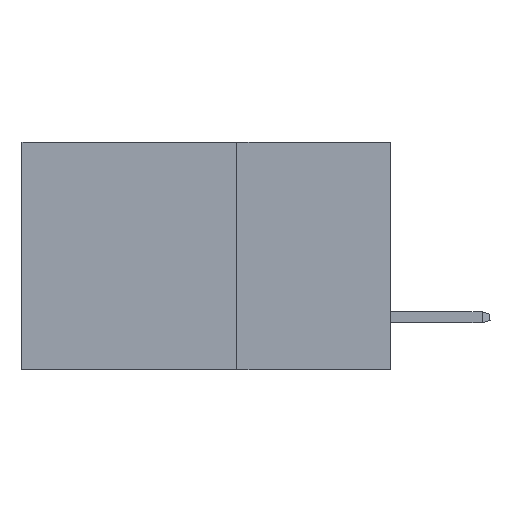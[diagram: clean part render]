
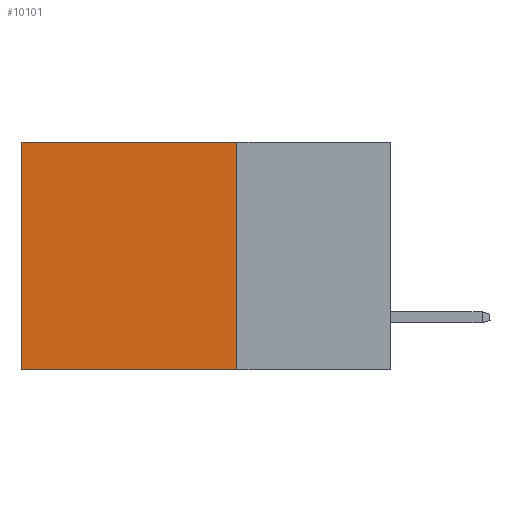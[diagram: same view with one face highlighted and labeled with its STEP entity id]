
A CAD part, left-side view. The second image highlights one B-rep face of the part: STEP entity #10101.
In plain terms, the highlighted planar face has unit normal (-1, 0, 0).
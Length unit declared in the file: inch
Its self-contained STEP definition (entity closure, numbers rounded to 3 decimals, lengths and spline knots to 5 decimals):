
#240 = ORIENTED_EDGE ( 'NONE', *, *, #2919, .T. ) ;
#477 = EDGE_LOOP ( 'NONE', ( #240, #1114, #8735, #3620 ) ) ;
#1114 = ORIENTED_EDGE ( 'NONE', *, *, #8586, .F. ) ;
#1245 = DIRECTION ( 'NONE',  ( 1., 0., 0. ) ) ;
#1264 = VECTOR ( 'NONE', #7803, 39.37008 ) ;
#1286 = PLANE ( 'NONE',  #10091 ) ;
#1387 = EDGE_CURVE ( 'NONE', #11843, #10115, #9545, .T. ) ;
#1590 = CARTESIAN_POINT ( 'NONE',  ( 0.2875, 0.25, -0.37 ) ) ;
#1961 = DIRECTION ( 'NONE',  ( 0., 0., -1. ) ) ;
#2145 = VERTEX_POINT ( 'NONE', #10215 ) ;
#2252 = DIRECTION ( 'NONE',  ( 0., 0., -1. ) ) ;
#2389 = CARTESIAN_POINT ( 'NONE',  ( 0.2875, 0.6, 0. ) ) ;
#2861 = CARTESIAN_POINT ( 'NONE',  ( 0.2875, 0.25, 0. ) ) ;
#2919 = EDGE_CURVE ( 'NONE', #10115, #2145, #11618, .T. ) ;
#3246 = CARTESIAN_POINT ( 'NONE',  ( 0.2875, 0.6, 0. ) ) ;
#3293 = LINE ( 'NONE', #2861, #10336 ) ;
#3432 = FACE_OUTER_BOUND ( 'NONE', #477, .T. ) ;
#3504 = DIRECTION ( 'NONE',  ( 0., 1., 0. ) ) ;
#3620 = ORIENTED_EDGE ( 'NONE', *, *, #1387, .T. ) ;
#4199 = CARTESIAN_POINT ( 'NONE',  ( 0.2875, 0.25, 0. ) ) ;
#4408 = CARTESIAN_POINT ( 'NONE',  ( 0.2875, 0.25, -0.37 ) ) ;
#4729 = LINE ( 'NONE', #1590, #10230 ) ;
#5136 = VERTEX_POINT ( 'NONE', #4408 ) ;
#5905 = VECTOR ( 'NONE', #10226, 39.37008 ) ;
#6294 = CARTESIAN_POINT ( 'NONE',  ( 0.2875, 0.25, 0. ) ) ;
#7803 = DIRECTION ( 'NONE',  ( 0., 0., -1. ) ) ;
#8372 = CARTESIAN_POINT ( 'NONE',  ( 0.2875, 0.25, 0. ) ) ;
#8586 = EDGE_CURVE ( 'NONE', #5136, #2145, #4729, .T. ) ;
#8735 = ORIENTED_EDGE ( 'NONE', *, *, #10522, .F. ) ;
#9545 = LINE ( 'NONE', #8372, #5905 ) ;
#10091 = AXIS2_PLACEMENT_3D ( 'NONE', #4199, #1245, #2252 ) ;
#10101 = ADVANCED_FACE ( 'NONE', ( #3432 ), #1286, .F. ) ;
#10115 = VERTEX_POINT ( 'NONE', #3246 ) ;
#10215 = CARTESIAN_POINT ( 'NONE',  ( 0.2875, 0.6, -0.37 ) ) ;
#10226 = DIRECTION ( 'NONE',  ( 0., 1., 0. ) ) ;
#10230 = VECTOR ( 'NONE', #3504, 39.37008 ) ;
#10336 = VECTOR ( 'NONE', #1961, 39.37008 ) ;
#10522 = EDGE_CURVE ( 'NONE', #11843, #5136, #3293, .T. ) ;
#11618 = LINE ( 'NONE', #2389, #1264 ) ;
#11843 = VERTEX_POINT ( 'NONE', #6294 ) ;
